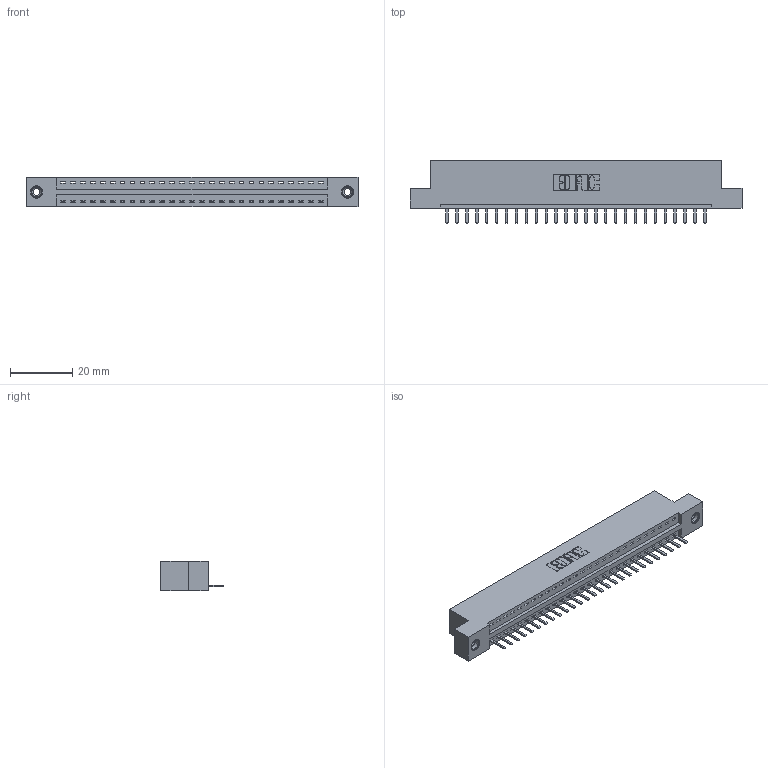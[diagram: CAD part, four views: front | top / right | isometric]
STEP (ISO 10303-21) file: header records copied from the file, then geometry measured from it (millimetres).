
FILE_DESCRIPTION (( 'STEP AP203' ), '1' );
FILE_NAME ('396-027-520-108.STEP', '2019-10-27T07:37:26', ( '' ), ( '' ), 'SwSTEP 2.0', 'SolidWorks 2016', '' );
FILE_SCHEMA (( 'CONFIG_CONTROL_DESIGN' ));
Length unit declared in the file: inch
Products named in the file (4): 345-292-001_345-293-120; 396-027-520-108; 345-250-001_345-250-003-102; 346 Part_Flush Mounting Lugs - 0.156 Dia-TI
Assembly tree (30 placements, depth 2):
  396-027-520-108
    346 Part_Flush Mounting Lugs - 0.156 Dia-TI
    345-292-001_345-293-120  x27
    345-250-001_345-250-003-102  x2
Bounding box: 106.3 x 20.02 x 9.4 mm (x, y, z)
Volume: 9987.6 mm3; surface area: 12083.9 mm2
Topology: 30 solids, 30 shells, 1856 faces, 5433 edges, 3542 vertices
Faces by surface type: plane 1242, cylinder 598, cone 12, torus 4
Entity records: 20076 total; most frequent: CARTESIAN_POINT 3440, ORIENTED_EDGE 3382, DIRECTION 3067, EDGE_CURVE 1691, LINE 1427, VECTOR 1427, VERTEX_POINT 1120, AXIS2_PLACEMENT_3D 820
